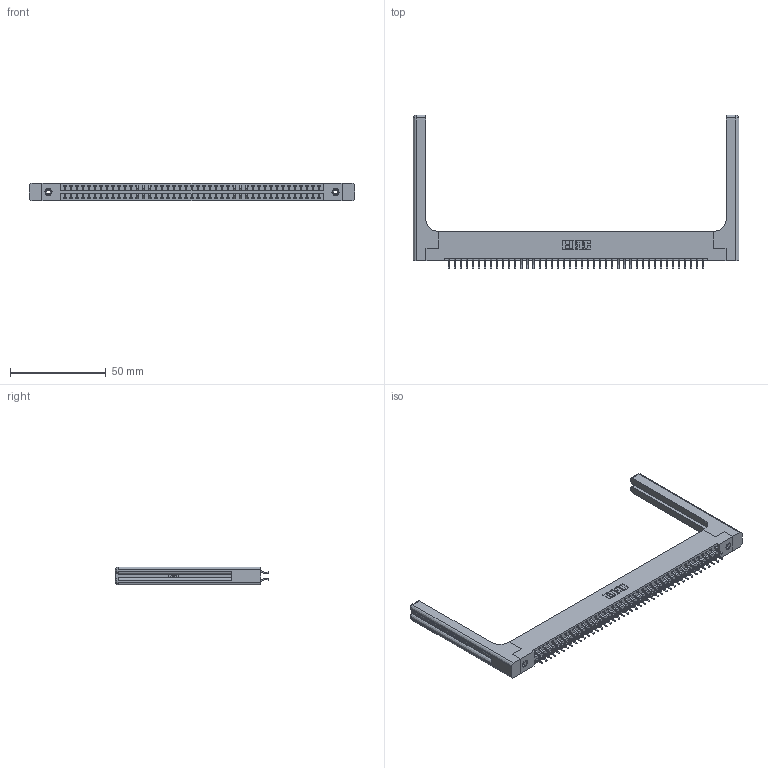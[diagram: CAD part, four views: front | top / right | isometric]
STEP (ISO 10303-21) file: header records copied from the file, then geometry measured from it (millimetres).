
FILE_DESCRIPTION (( 'STEP AP203' ), '1' );
FILE_NAME ('346-086-556-258.STEP', '2022-05-25T23:10:20', ( '' ), ( '' ), 'SwSTEP 2.0', 'SolidWorks 2020', '' );
FILE_SCHEMA (( 'CONFIG_CONTROL_DESIGN' ));
Length unit declared in the file: inch
Products named in the file (5): 345-292-001_556 Tail; 345-250-001_345-250-001-102; 346 Part_Flush Mounting Lugs - 0.156 Dia-TH; 346-220-058_345-220-058; 346-086-556-258
Assembly tree (91 placements, depth 2):
  346-086-556-258
    346 Part_Flush Mounting Lugs - 0.156 Dia-TH
    345-292-001_556 Tail  x86
    345-250-001_345-250-001-102  x2
    346-220-058_345-220-058  x2
Bounding box: 170.59 x 80.53 x 9.4 mm (x, y, z)
Volume: 20092 mm3; surface area: 35985 mm2
Topology: 91 solids, 91 shells, 5380 faces, 15884 edges, 10470 vertices
Faces by surface type: plane 3592, cylinder 1728, bspline 36, cone 12, sphere 8, torus 4
Full cylindrical faces by diameter (mm): 0.349 x6, 0.499 x22, 1.334 x3, 1.575 x2, 1.596 x6, 1.626 x1, 2.032 x84, 3.962 x1
Entity records: 33746 total; most frequent: CARTESIAN_POINT 6587, ORIENTED_EDGE 5304, DIRECTION 4776, EDGE_CURVE 2652, LINE 2248, VECTOR 2248, VERTEX_POINT 1758, AXIS2_PLACEMENT_3D 1264
